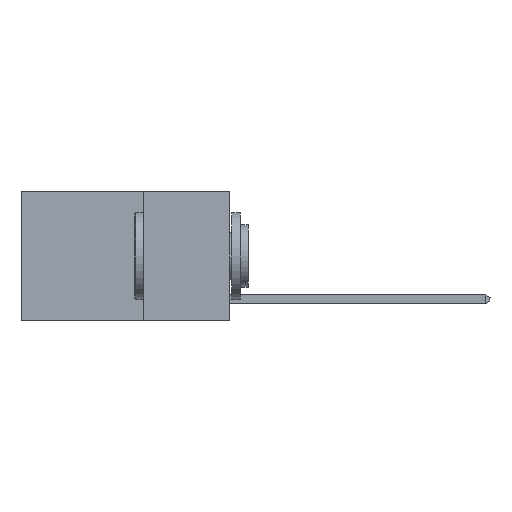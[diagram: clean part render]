
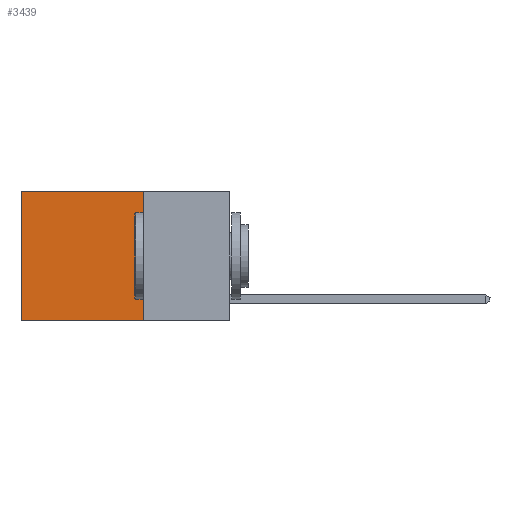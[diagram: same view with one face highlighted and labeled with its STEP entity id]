
A CAD part, left-side view. The second image highlights one B-rep face of the part: STEP entity #3439.
In plain terms, the highlighted planar face has unit normal (-1, 0, 0).
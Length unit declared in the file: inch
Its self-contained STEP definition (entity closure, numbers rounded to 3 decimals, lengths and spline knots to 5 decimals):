
#33 = ORIENTED_EDGE ( 'NONE', *, *, #10042, .T. ) ;
#407 = LINE ( 'NONE', #11825, #14145 ) ;
#758 = LINE ( 'NONE', #18756, #5837 ) ;
#807 = DIRECTION ( 'NONE',  ( 1., 0., 0. ) ) ;
#3093 = PLANE ( 'NONE',  #27749 ) ;
#3439 = ADVANCED_FACE ( 'NONE', ( #21387 ), #3093, .F. ) ;
#3525 = VERTEX_POINT ( 'NONE', #23820 ) ;
#4282 = VERTEX_POINT ( 'NONE', #10127 ) ;
#5837 = VECTOR ( 'NONE', #16486, 39.37008 ) ;
#8422 = CARTESIAN_POINT ( 'NONE',  ( 0.2625, 0.25, -0.37 ) ) ;
#9440 = VERTEX_POINT ( 'NONE', #16315 ) ;
#10042 = EDGE_CURVE ( 'NONE', #9440, #28883, #407, .T. ) ;
#10127 = CARTESIAN_POINT ( 'NONE',  ( 0.2625, 0.25, -0.37 ) ) ;
#10139 = VECTOR ( 'NONE', #29666, 39.37008 ) ;
#11673 = DIRECTION ( 'NONE',  ( 0., 0., -1. ) ) ;
#11825 = CARTESIAN_POINT ( 'NONE',  ( 0.2625, 0.6, 0. ) ) ;
#12086 = CARTESIAN_POINT ( 'NONE',  ( 0.2625, 0.25, 0. ) ) ;
#12389 = DIRECTION ( 'NONE',  ( 0., 0., -1. ) ) ;
#13403 = LINE ( 'NONE', #20412, #10139 ) ;
#14145 = VECTOR ( 'NONE', #11673, 39.37008 ) ;
#14561 = ORIENTED_EDGE ( 'NONE', *, *, #19667, .F. ) ;
#16315 = CARTESIAN_POINT ( 'NONE',  ( 0.2625, 0.6, 0. ) ) ;
#16486 = DIRECTION ( 'NONE',  ( 0., 1., 0. ) ) ;
#16560 = EDGE_LOOP ( 'NONE', ( #33, #14561, #29670, #29572 ) ) ;
#17368 = VECTOR ( 'NONE', #26702, 39.37008 ) ;
#18756 = CARTESIAN_POINT ( 'NONE',  ( 0.2625, 0.25, 0. ) ) ;
#19540 = CARTESIAN_POINT ( 'NONE',  ( 0.2625, 0.6, -0.37 ) ) ;
#19667 = EDGE_CURVE ( 'NONE', #4282, #28883, #27408, .T. ) ;
#20412 = CARTESIAN_POINT ( 'NONE',  ( 0.2625, 0.25, 0. ) ) ;
#21387 = FACE_OUTER_BOUND ( 'NONE', #16560, .T. ) ;
#22275 = EDGE_CURVE ( 'NONE', #3525, #9440, #758, .T. ) ;
#23820 = CARTESIAN_POINT ( 'NONE',  ( 0.2625, 0.25, 0. ) ) ;
#23860 = EDGE_CURVE ( 'NONE', #3525, #4282, #13403, .T. ) ;
#26702 = DIRECTION ( 'NONE',  ( 0., 1., 0. ) ) ;
#27408 = LINE ( 'NONE', #8422, #17368 ) ;
#27749 = AXIS2_PLACEMENT_3D ( 'NONE', #12086, #807, #12389 ) ;
#28883 = VERTEX_POINT ( 'NONE', #19540 ) ;
#29572 = ORIENTED_EDGE ( 'NONE', *, *, #22275, .T. ) ;
#29666 = DIRECTION ( 'NONE',  ( 0., 0., -1. ) ) ;
#29670 = ORIENTED_EDGE ( 'NONE', *, *, #23860, .F. ) ;
